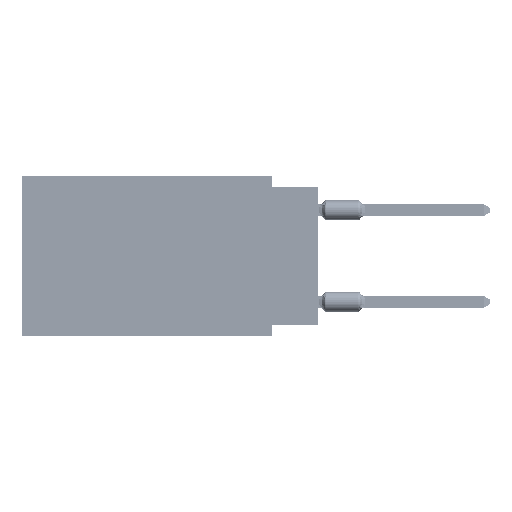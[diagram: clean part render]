
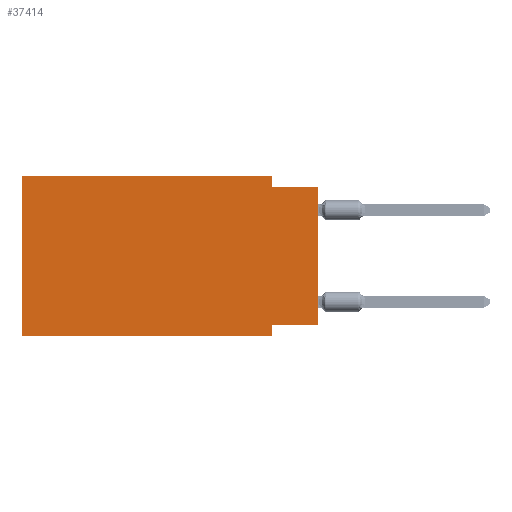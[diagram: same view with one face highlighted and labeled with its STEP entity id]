
A CAD part, left-side view. The second image highlights one B-rep face of the part: STEP entity #37414.
In plain terms, the highlighted planar face has unit normal (-1, 0, 0).
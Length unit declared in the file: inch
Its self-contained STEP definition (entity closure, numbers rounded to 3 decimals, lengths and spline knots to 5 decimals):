
#676 = EDGE_CURVE ( 'NONE', #55807, #87711, #30874, .T. ) ;
#2905 = ORIENTED_EDGE ( 'NONE', *, *, #11434, .F. ) ;
#4335 = PLANE ( 'NONE',  #29232 ) ;
#4801 = CARTESIAN_POINT ( 'NONE',  ( 0., 0.645, 0. ) ) ;
#5838 = EDGE_CURVE ( 'NONE', #106039, #114446, #48884, .T. ) ;
#6126 = CARTESIAN_POINT ( 'NONE',  ( 0., 0.645, 0. ) ) ;
#6318 = VERTEX_POINT ( 'NONE', #30647 ) ;
#8054 = ORIENTED_EDGE ( 'NONE', *, *, #96620, .F. ) ;
#9695 = ORIENTED_EDGE ( 'NONE', *, *, #83212, .F. ) ;
#11434 = EDGE_CURVE ( 'NONE', #106039, #33285, #81648, .T. ) ;
#12491 = EDGE_LOOP ( 'NONE', ( #73361, #50616, #79782, #8054, #9695, #93495, #80301, #2905 ) ) ;
#19002 = CARTESIAN_POINT ( 'NONE',  ( 0., 0., -0.325 ) ) ;
#19028 = CARTESIAN_POINT ( 'NONE',  ( 0., 0.1, 0. ) ) ;
#19217 = VECTOR ( 'NONE', #110320, 39.37008 ) ;
#20677 = CARTESIAN_POINT ( 'NONE',  ( 0., 0.645, 0. ) ) ;
#22569 = DIRECTION ( 'NONE',  ( 0., 1., 0. ) ) ;
#22913 = CARTESIAN_POINT ( 'NONE',  ( 0., 0.1, -0.35 ) ) ;
#27393 = LINE ( 'NONE', #100448, #43202 ) ;
#29232 = AXIS2_PLACEMENT_3D ( 'NONE', #20677, #75020, #30021 ) ;
#30021 = DIRECTION ( 'NONE',  ( 0., 0., -1. ) ) ;
#30647 = CARTESIAN_POINT ( 'NONE',  ( 0., 0.645, -0.35 ) ) ;
#30874 = LINE ( 'NONE', #66517, #96765 ) ;
#32113 = VECTOR ( 'NONE', #94758, 39.37008 ) ;
#33059 = VECTOR ( 'NONE', #60550, 39.37008 ) ;
#33285 = VERTEX_POINT ( 'NONE', #39601 ) ;
#34114 = LINE ( 'NONE', #6126, #98364 ) ;
#37414 = ADVANCED_FACE ( 'NONE', ( #92008 ), #4335, .F. ) ;
#39601 = CARTESIAN_POINT ( 'NONE',  ( 0., 0.1, -0.325 ) ) ;
#42176 = CARTESIAN_POINT ( 'NONE',  ( 0., 0.645, 0. ) ) ;
#43202 = VECTOR ( 'NONE', #56008, 39.37008 ) ;
#44725 = EDGE_CURVE ( 'NONE', #6318, #83246, #27393, .T. ) ;
#48627 = LINE ( 'NONE', #22913, #115515 ) ;
#48884 = LINE ( 'NONE', #93911, #19217 ) ;
#50616 = ORIENTED_EDGE ( 'NONE', *, *, #85477, .F. ) ;
#55807 = VERTEX_POINT ( 'NONE', #19028 ) ;
#56008 = DIRECTION ( 'NONE',  ( 0., -1., 0. ) ) ;
#59889 = EDGE_CURVE ( 'NONE', #33285, #83246, #48627, .T. ) ;
#60550 = DIRECTION ( 'NONE',  ( 0., -1., 0. ) ) ;
#65821 = CARTESIAN_POINT ( 'NONE',  ( 0., 0., -0.325 ) ) ;
#66517 = CARTESIAN_POINT ( 'NONE',  ( 0., 0.1, 0. ) ) ;
#69766 = DIRECTION ( 'NONE',  ( 0., 0., 1. ) ) ;
#73361 = ORIENTED_EDGE ( 'NONE', *, *, #5838, .T. ) ;
#75020 = DIRECTION ( 'NONE',  ( 1., 0., 0. ) ) ;
#78652 = CARTESIAN_POINT ( 'NONE',  ( 0., 0., -0.025 ) ) ;
#79782 = ORIENTED_EDGE ( 'NONE', *, *, #676, .F. ) ;
#80301 = ORIENTED_EDGE ( 'NONE', *, *, #59889, .F. ) ;
#81648 = LINE ( 'NONE', #65821, #110928 ) ;
#82272 = VERTEX_POINT ( 'NONE', #42176 ) ;
#83212 = EDGE_CURVE ( 'NONE', #6318, #82272, #34114, .T. ) ;
#83246 = VERTEX_POINT ( 'NONE', #103187 ) ;
#84853 = LINE ( 'NONE', #4801, #32113 ) ;
#85477 = EDGE_CURVE ( 'NONE', #87711, #114446, #106759, .T. ) ;
#87711 = VERTEX_POINT ( 'NONE', #99393 ) ;
#92008 = FACE_OUTER_BOUND ( 'NONE', #12491, .T. ) ;
#92285 = DIRECTION ( 'NONE',  ( 0., 0., -1. ) ) ;
#93495 = ORIENTED_EDGE ( 'NONE', *, *, #44725, .T. ) ;
#93911 = CARTESIAN_POINT ( 'NONE',  ( 0., 0., 0. ) ) ;
#94758 = DIRECTION ( 'NONE',  ( 0., -1., 0. ) ) ;
#96620 = EDGE_CURVE ( 'NONE', #82272, #55807, #84853, .T. ) ;
#96765 = VECTOR ( 'NONE', #92285, 39.37008 ) ;
#98364 = VECTOR ( 'NONE', #69766, 39.37008 ) ;
#99393 = CARTESIAN_POINT ( 'NONE',  ( 0., 0.1, -0.025 ) ) ;
#100448 = CARTESIAN_POINT ( 'NONE',  ( 0., 0.645, -0.35 ) ) ;
#103017 = DIRECTION ( 'NONE',  ( 0., 0., -1. ) ) ;
#103187 = CARTESIAN_POINT ( 'NONE',  ( 0., 0.1, -0.35 ) ) ;
#106039 = VERTEX_POINT ( 'NONE', #19002 ) ;
#106759 = LINE ( 'NONE', #78652, #33059 ) ;
#110320 = DIRECTION ( 'NONE',  ( 0., 0., 1. ) ) ;
#110928 = VECTOR ( 'NONE', #22569, 39.37008 ) ;
#114446 = VERTEX_POINT ( 'NONE', #115050 ) ;
#115050 = CARTESIAN_POINT ( 'NONE',  ( 0., 0., -0.025 ) ) ;
#115515 = VECTOR ( 'NONE', #103017, 39.37008 ) ;
